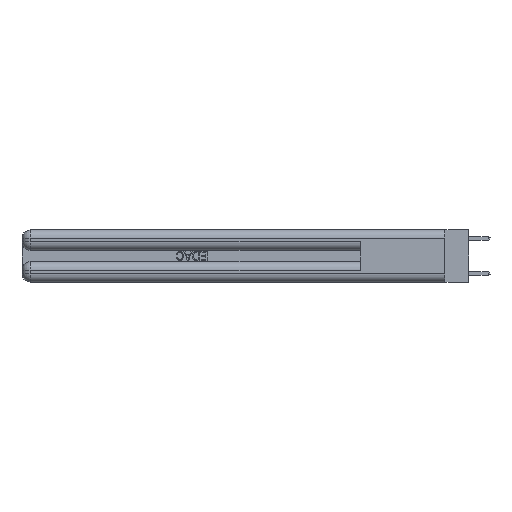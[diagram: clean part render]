
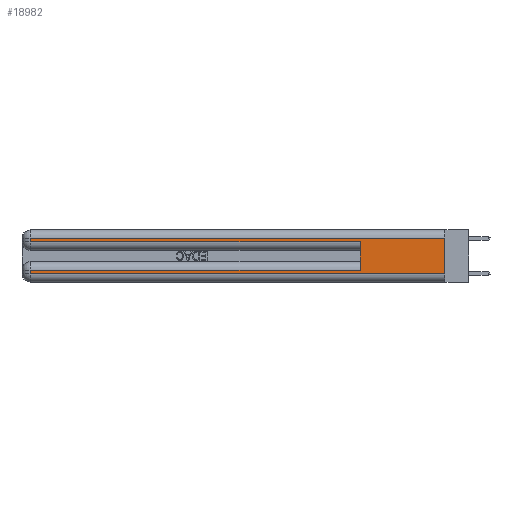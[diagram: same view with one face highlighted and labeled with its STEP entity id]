
A CAD part, left-side view. The second image highlights one B-rep face of the part: STEP entity #18982.
In plain terms, the highlighted planar face has unit normal (-1, 0, 0).
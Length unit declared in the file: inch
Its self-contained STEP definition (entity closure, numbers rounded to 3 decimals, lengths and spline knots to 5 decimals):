
#937 = AXIS2_PLACEMENT_3D ( 'NONE', #5296, #21599, #7987 ) ;
#1178 = DIRECTION ( 'NONE',  ( 0., -1., 0. ) ) ;
#1244 = PLANE ( 'NONE',  #937 ) ;
#1344 = EDGE_CURVE ( 'NONE', #13835, #16591, #6176, .T. ) ;
#1484 = VECTOR ( 'NONE', #1178, 39.37008 ) ;
#2345 = DIRECTION ( 'NONE',  ( 0., 1., 0. ) ) ;
#2458 = EDGE_CURVE ( 'NONE', #18723, #15275, #6811, .T. ) ;
#2758 = DIRECTION ( 'NONE',  ( 0., 0., -1. ) ) ;
#2918 = VECTOR ( 'NONE', #23503, 39.37008 ) ;
#3082 = VECTOR ( 'NONE', #2345, 39.37008 ) ;
#3157 = ORIENTED_EDGE ( 'NONE', *, *, #26041, .F. ) ;
#3418 = CARTESIAN_POINT ( 'NONE',  ( 0., 0., 0.06 ) ) ;
#3558 = CARTESIAN_POINT ( 'NONE',  ( 0., 0., 0.31 ) ) ;
#4704 = VECTOR ( 'NONE', #15866, 39.37008 ) ;
#5296 = CARTESIAN_POINT ( 'NONE',  ( 0., 0., 0.37 ) ) ;
#5837 = ORIENTED_EDGE ( 'NONE', *, *, #15967, .T. ) ;
#5881 = CARTESIAN_POINT ( 'NONE',  ( 0., 2.94, 0.37 ) ) ;
#6097 = LINE ( 'NONE', #3418, #1484 ) ;
#6176 = LINE ( 'NONE', #5881, #10083 ) ;
#6723 = EDGE_CURVE ( 'NONE', #25188, #13835, #18514, .T. ) ;
#6753 = LINE ( 'NONE', #13305, #4704 ) ;
#6811 = LINE ( 'NONE', #18182, #9974 ) ;
#7116 = CARTESIAN_POINT ( 'NONE',  ( 0., 2.94, 0.37 ) ) ;
#7987 = DIRECTION ( 'NONE',  ( 0., 0., -1. ) ) ;
#9860 = EDGE_CURVE ( 'NONE', #25188, #15275, #20266, .T. ) ;
#9974 = VECTOR ( 'NONE', #27748, 39.37008 ) ;
#10083 = VECTOR ( 'NONE', #22322, 39.37008 ) ;
#10232 = CARTESIAN_POINT ( 'NONE',  ( 0., 0., 0.06 ) ) ;
#10339 = CARTESIAN_POINT ( 'NONE',  ( 0., 0., 0.37 ) ) ;
#10930 = CARTESIAN_POINT ( 'NONE',  ( 0., 0.6, 0.085 ) ) ;
#11269 = CARTESIAN_POINT ( 'NONE',  ( 0., 2.94, 0.285 ) ) ;
#11762 = ORIENTED_EDGE ( 'NONE', *, *, #9860, .F. ) ;
#12048 = ORIENTED_EDGE ( 'NONE', *, *, #2458, .T. ) ;
#13305 = CARTESIAN_POINT ( 'NONE',  ( 0., 0., 0.31 ) ) ;
#13835 = VERTEX_POINT ( 'NONE', #28197 ) ;
#14579 = ORIENTED_EDGE ( 'NONE', *, *, #6723, .T. ) ;
#15275 = VERTEX_POINT ( 'NONE', #21369 ) ;
#15866 = DIRECTION ( 'NONE',  ( 0., 1., 0. ) ) ;
#15967 = EDGE_CURVE ( 'NONE', #20117, #23182, #6753, .T. ) ;
#16385 = VECTOR ( 'NONE', #26542, 39.37008 ) ;
#16591 = VERTEX_POINT ( 'NONE', #18235 ) ;
#17217 = VECTOR ( 'NONE', #2758, 39.37008 ) ;
#18182 = CARTESIAN_POINT ( 'NONE',  ( 0., 0., 0.285 ) ) ;
#18235 = CARTESIAN_POINT ( 'NONE',  ( 0., 2.94, 0.06 ) ) ;
#18327 = LINE ( 'NONE', #7116, #17217 ) ;
#18514 = LINE ( 'NONE', #21053, #3082 ) ;
#18723 = VERTEX_POINT ( 'NONE', #11269 ) ;
#18982 = ADVANCED_FACE ( 'NONE', ( #23973 ), #1244, .F. ) ;
#20117 = VERTEX_POINT ( 'NONE', #3558 ) ;
#20197 = EDGE_CURVE ( 'NONE', #23182, #18723, #18327, .T. ) ;
#20266 = LINE ( 'NONE', #29224, #16385 ) ;
#21053 = CARTESIAN_POINT ( 'NONE',  ( 0., 0., 0.085 ) ) ;
#21106 = EDGE_CURVE ( 'NONE', #16591, #21984, #6097, .T. ) ;
#21369 = CARTESIAN_POINT ( 'NONE',  ( 0., 0.6, 0.285 ) ) ;
#21599 = DIRECTION ( 'NONE',  ( 1., 0., 0. ) ) ;
#21984 = VERTEX_POINT ( 'NONE', #10232 ) ;
#22322 = DIRECTION ( 'NONE',  ( 0., 0., -1. ) ) ;
#22986 = ORIENTED_EDGE ( 'NONE', *, *, #20197, .T. ) ;
#23182 = VERTEX_POINT ( 'NONE', #25810 ) ;
#23503 = DIRECTION ( 'NONE',  ( 0., 0., -1. ) ) ;
#23973 = FACE_OUTER_BOUND ( 'NONE', #24578, .T. ) ;
#24225 = ORIENTED_EDGE ( 'NONE', *, *, #21106, .T. ) ;
#24578 = EDGE_LOOP ( 'NONE', ( #3157, #5837, #22986, #12048, #11762, #14579, #28040, #24225 ) ) ;
#25188 = VERTEX_POINT ( 'NONE', #10930 ) ;
#25810 = CARTESIAN_POINT ( 'NONE',  ( 0., 2.94, 0.31 ) ) ;
#25915 = LINE ( 'NONE', #10339, #2918 ) ;
#26041 = EDGE_CURVE ( 'NONE', #20117, #21984, #25915, .T. ) ;
#26542 = DIRECTION ( 'NONE',  ( 0., 0., 1. ) ) ;
#27748 = DIRECTION ( 'NONE',  ( 0., -1., 0. ) ) ;
#28040 = ORIENTED_EDGE ( 'NONE', *, *, #1344, .T. ) ;
#28197 = CARTESIAN_POINT ( 'NONE',  ( 0., 2.94, 0.085 ) ) ;
#29224 = CARTESIAN_POINT ( 'NONE',  ( 0., 0.6, 0.145 ) ) ;
